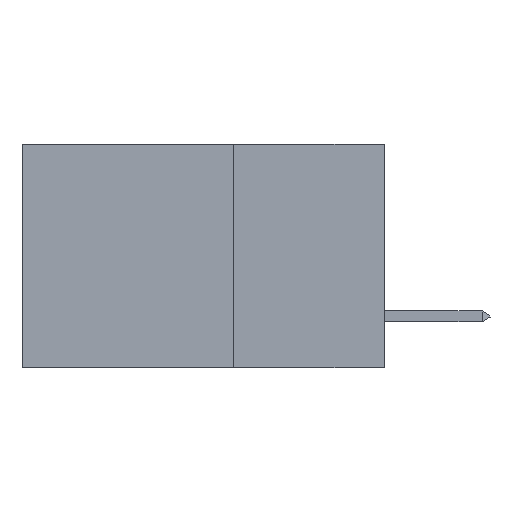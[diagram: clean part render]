
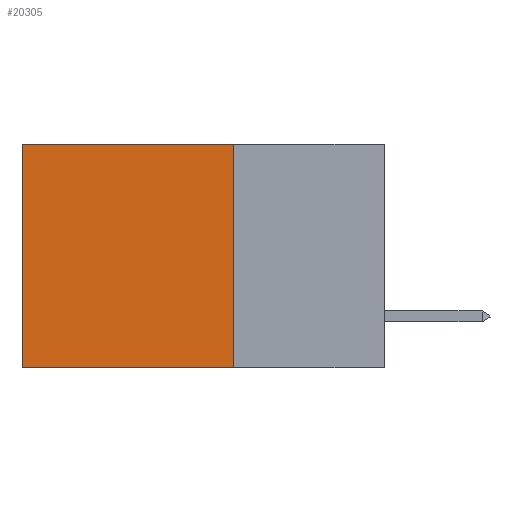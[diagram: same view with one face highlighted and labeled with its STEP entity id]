
A CAD part, left-side view. The second image highlights one B-rep face of the part: STEP entity #20305.
In plain terms, the highlighted planar face has unit normal (-1, 0, 0).
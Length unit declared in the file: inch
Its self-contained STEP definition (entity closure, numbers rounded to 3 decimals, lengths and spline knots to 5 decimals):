
#2045 = LINE ( 'NONE', #5597, #3434 ) ;
#3259 = VERTEX_POINT ( 'NONE', #24801 ) ;
#3434 = VECTOR ( 'NONE', #3449, 39.37008 ) ;
#3449 = DIRECTION ( 'NONE',  ( 0., 0., -1. ) ) ;
#3611 = AXIS2_PLACEMENT_3D ( 'NONE', #22749, #15914, #27590 ) ;
#4297 = ORIENTED_EDGE ( 'NONE', *, *, #28612, .T. ) ;
#4327 = CARTESIAN_POINT ( 'NONE',  ( 0.2875, 0.25, 0. ) ) ;
#5556 = VECTOR ( 'NONE', #18251, 39.37008 ) ;
#5597 = CARTESIAN_POINT ( 'NONE',  ( 0.2875, 0.6, 0. ) ) ;
#6956 = LINE ( 'NONE', #7201, #5556 ) ;
#7201 = CARTESIAN_POINT ( 'NONE',  ( 0.2875, 0.25, 0. ) ) ;
#7453 = CARTESIAN_POINT ( 'NONE',  ( 0.2875, 0.25, -0.37 ) ) ;
#9640 = FACE_OUTER_BOUND ( 'NONE', #13854, .T. ) ;
#11270 = ORIENTED_EDGE ( 'NONE', *, *, #11655, .F. ) ;
#11329 = VECTOR ( 'NONE', #16532, 39.37008 ) ;
#11655 = EDGE_CURVE ( 'NONE', #18256, #28707, #13466, .T. ) ;
#12945 = VECTOR ( 'NONE', #13460, 39.37008 ) ;
#13460 = DIRECTION ( 'NONE',  ( 0., 1., 0. ) ) ;
#13466 = LINE ( 'NONE', #7453, #11329 ) ;
#13854 = EDGE_LOOP ( 'NONE', ( #4297, #11270, #26350, #27605 ) ) ;
#15205 = EDGE_CURVE ( 'NONE', #3259, #16845, #18860, .T. ) ;
#15914 = DIRECTION ( 'NONE',  ( 1., 0., 0. ) ) ;
#16532 = DIRECTION ( 'NONE',  ( 0., 1., 0. ) ) ;
#16845 = VERTEX_POINT ( 'NONE', #20738 ) ;
#18069 = PLANE ( 'NONE',  #3611 ) ;
#18251 = DIRECTION ( 'NONE',  ( 0., 0., -1. ) ) ;
#18256 = VERTEX_POINT ( 'NONE', #20533 ) ;
#18860 = LINE ( 'NONE', #4327, #12945 ) ;
#19412 = CARTESIAN_POINT ( 'NONE',  ( 0.2875, 0.6, -0.37 ) ) ;
#20305 = ADVANCED_FACE ( 'NONE', ( #9640 ), #18069, .F. ) ;
#20533 = CARTESIAN_POINT ( 'NONE',  ( 0.2875, 0.25, -0.37 ) ) ;
#20738 = CARTESIAN_POINT ( 'NONE',  ( 0.2875, 0.6, 0. ) ) ;
#22749 = CARTESIAN_POINT ( 'NONE',  ( 0.2875, 0.25, 0. ) ) ;
#24801 = CARTESIAN_POINT ( 'NONE',  ( 0.2875, 0.25, 0. ) ) ;
#26350 = ORIENTED_EDGE ( 'NONE', *, *, #28095, .F. ) ;
#27590 = DIRECTION ( 'NONE',  ( 0., 0., -1. ) ) ;
#27605 = ORIENTED_EDGE ( 'NONE', *, *, #15205, .T. ) ;
#28095 = EDGE_CURVE ( 'NONE', #3259, #18256, #6956, .T. ) ;
#28612 = EDGE_CURVE ( 'NONE', #16845, #28707, #2045, .T. ) ;
#28707 = VERTEX_POINT ( 'NONE', #19412 ) ;
